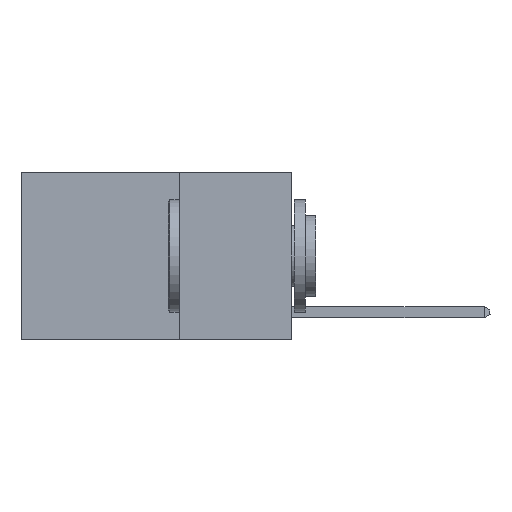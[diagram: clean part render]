
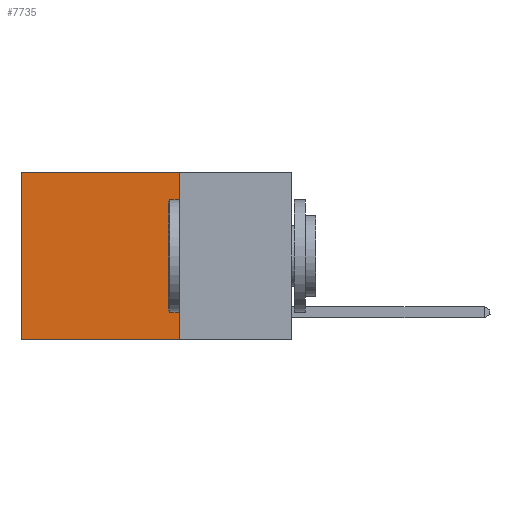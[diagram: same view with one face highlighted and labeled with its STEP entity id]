
A CAD part, left-side view. The second image highlights one B-rep face of the part: STEP entity #7735.
In plain terms, the highlighted planar face has unit normal (-1, 0, 0).
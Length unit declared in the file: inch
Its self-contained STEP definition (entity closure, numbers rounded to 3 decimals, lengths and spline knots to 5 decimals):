
#89 = VECTOR ( 'NONE', #15099, 39.37008 ) ;
#1874 = LINE ( 'NONE', #9217, #7688 ) ;
#1996 = DIRECTION ( 'NONE',  ( 0., 1., 0. ) ) ;
#2868 = ORIENTED_EDGE ( 'NONE', *, *, #18096, .T. ) ;
#3107 = VERTEX_POINT ( 'NONE', #5788 ) ;
#4027 = ORIENTED_EDGE ( 'NONE', *, *, #22750, .T. ) ;
#4179 = PLANE ( 'NONE',  #6422 ) ;
#4297 = CARTESIAN_POINT ( 'NONE',  ( 0.2625, 0.25, 0. ) ) ;
#5281 = DIRECTION ( 'NONE',  ( 0., 0., -1. ) ) ;
#5359 = VECTOR ( 'NONE', #5281, 39.37008 ) ;
#5788 = CARTESIAN_POINT ( 'NONE',  ( 0.2625, 0.6, -0.37 ) ) ;
#6183 = CARTESIAN_POINT ( 'NONE',  ( 0.2625, 0.25, -0.37 ) ) ;
#6422 = AXIS2_PLACEMENT_3D ( 'NONE', #22700, #22813, #20519 ) ;
#7688 = VECTOR ( 'NONE', #1996, 39.37008 ) ;
#7735 = ADVANCED_FACE ( 'NONE', ( #9713 ), #4179, .F. ) ;
#8575 = DIRECTION ( 'NONE',  ( 0., 0., -1. ) ) ;
#9217 = CARTESIAN_POINT ( 'NONE',  ( 0.2625, 0.25, -0.37 ) ) ;
#9713 = FACE_OUTER_BOUND ( 'NONE', #21728, .T. ) ;
#10284 = EDGE_CURVE ( 'NONE', #16994, #18533, #15964, .T. ) ;
#10932 = EDGE_CURVE ( 'NONE', #18533, #3107, #1874, .T. ) ;
#12040 = LINE ( 'NONE', #17427, #22478 ) ;
#14007 = VERTEX_POINT ( 'NONE', #15068 ) ;
#15068 = CARTESIAN_POINT ( 'NONE',  ( 0.2625, 0.6, 0. ) ) ;
#15099 = DIRECTION ( 'NONE',  ( 0., 1., 0. ) ) ;
#15964 = LINE ( 'NONE', #19707, #5359 ) ;
#16994 = VERTEX_POINT ( 'NONE', #18698 ) ;
#17427 = CARTESIAN_POINT ( 'NONE',  ( 0.2625, 0.6, 0. ) ) ;
#18096 = EDGE_CURVE ( 'NONE', #16994, #14007, #20759, .T. ) ;
#18533 = VERTEX_POINT ( 'NONE', #6183 ) ;
#18698 = CARTESIAN_POINT ( 'NONE',  ( 0.2625, 0.25, 0. ) ) ;
#18792 = ORIENTED_EDGE ( 'NONE', *, *, #10932, .F. ) ;
#19707 = CARTESIAN_POINT ( 'NONE',  ( 0.2625, 0.25, 0. ) ) ;
#20519 = DIRECTION ( 'NONE',  ( 0., 0., -1. ) ) ;
#20759 = LINE ( 'NONE', #4297, #89 ) ;
#21728 = EDGE_LOOP ( 'NONE', ( #4027, #18792, #22837, #2868 ) ) ;
#22478 = VECTOR ( 'NONE', #8575, 39.37008 ) ;
#22700 = CARTESIAN_POINT ( 'NONE',  ( 0.2625, 0.25, 0. ) ) ;
#22750 = EDGE_CURVE ( 'NONE', #14007, #3107, #12040, .T. ) ;
#22813 = DIRECTION ( 'NONE',  ( 1., 0., 0. ) ) ;
#22837 = ORIENTED_EDGE ( 'NONE', *, *, #10284, .F. ) ;
